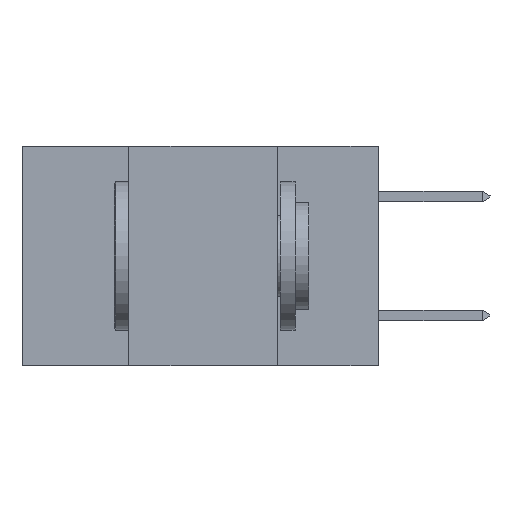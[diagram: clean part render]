
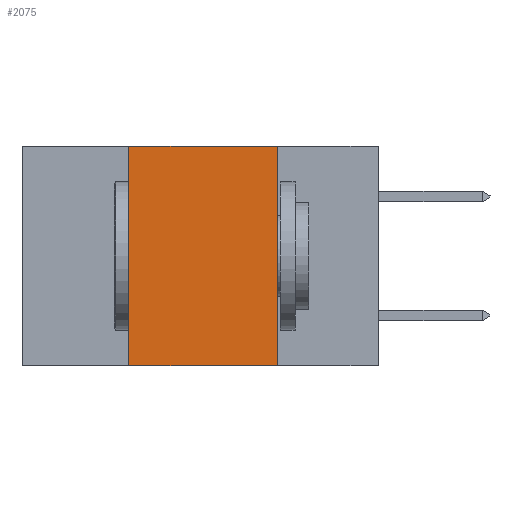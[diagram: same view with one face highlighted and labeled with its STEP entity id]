
A CAD part, left-side view. The second image highlights one B-rep face of the part: STEP entity #2075.
In plain terms, the highlighted planar face has unit normal (-1, 0, 0).
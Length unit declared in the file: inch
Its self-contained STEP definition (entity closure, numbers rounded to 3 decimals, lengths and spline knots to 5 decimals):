
#1141 = CARTESIAN_POINT ( 'NONE',  ( 0., 0.17, -0.37 ) ) ;
#2075 = ADVANCED_FACE ( 'NONE', ( #20528 ), #10109, .F. ) ;
#2426 = VECTOR ( 'NONE', #7298, 39.37008 ) ;
#3130 = CARTESIAN_POINT ( 'NONE',  ( 0., 0.6, 0. ) ) ;
#3871 = CARTESIAN_POINT ( 'NONE',  ( 0., 0.6, -0.37 ) ) ;
#3981 = LINE ( 'NONE', #3871, #6987 ) ;
#5074 = LINE ( 'NONE', #1141, #17252 ) ;
#5082 = LINE ( 'NONE', #11952, #12541 ) ;
#6987 = VECTOR ( 'NONE', #17351, 39.37008 ) ;
#7298 = DIRECTION ( 'NONE',  ( 0., -1., 0. ) ) ;
#7911 = ORIENTED_EDGE ( 'NONE', *, *, #15079, .T. ) ;
#8252 = CARTESIAN_POINT ( 'NONE',  ( 0., 0.42, -0.37 ) ) ;
#9280 = CARTESIAN_POINT ( 'NONE',  ( 0., 0.17, -0.37 ) ) ;
#9911 = CARTESIAN_POINT ( 'NONE',  ( 0., 0.42, 0. ) ) ;
#9912 = ORIENTED_EDGE ( 'NONE', *, *, #12412, .F. ) ;
#10005 = DIRECTION ( 'NONE',  ( 1., 0., 0. ) ) ;
#10109 = PLANE ( 'NONE',  #20768 ) ;
#10764 = VERTEX_POINT ( 'NONE', #8252 ) ;
#11936 = EDGE_CURVE ( 'NONE', #15763, #19973, #20974, .T. ) ;
#11952 = CARTESIAN_POINT ( 'NONE',  ( 0., 0.42, -0.37 ) ) ;
#12412 = EDGE_CURVE ( 'NONE', #19973, #20017, #5074, .T. ) ;
#12541 = VECTOR ( 'NONE', #18881, 39.37008 ) ;
#15079 = EDGE_CURVE ( 'NONE', #10764, #20017, #3981, .T. ) ;
#15763 = VERTEX_POINT ( 'NONE', #9911 ) ;
#16712 = DIRECTION ( 'NONE',  ( 0., 0., -1. ) ) ;
#16836 = ORIENTED_EDGE ( 'NONE', *, *, #16854, .F. ) ;
#16854 = EDGE_CURVE ( 'NONE', #10764, #15763, #5082, .T. ) ;
#17252 = VECTOR ( 'NONE', #20558, 39.37008 ) ;
#17351 = DIRECTION ( 'NONE',  ( 0., -1., 0. ) ) ;
#17620 = CARTESIAN_POINT ( 'NONE',  ( 0., 0.6, 0. ) ) ;
#17798 = CARTESIAN_POINT ( 'NONE',  ( 0., 0.17, 0. ) ) ;
#18144 = ORIENTED_EDGE ( 'NONE', *, *, #11936, .F. ) ;
#18881 = DIRECTION ( 'NONE',  ( 0., 0., 1. ) ) ;
#19973 = VERTEX_POINT ( 'NONE', #17798 ) ;
#20017 = VERTEX_POINT ( 'NONE', #9280 ) ;
#20528 = FACE_OUTER_BOUND ( 'NONE', #20686, .T. ) ;
#20558 = DIRECTION ( 'NONE',  ( 0., 0., -1. ) ) ;
#20686 = EDGE_LOOP ( 'NONE', ( #9912, #18144, #16836, #7911 ) ) ;
#20768 = AXIS2_PLACEMENT_3D ( 'NONE', #3130, #10005, #16712 ) ;
#20974 = LINE ( 'NONE', #17620, #2426 ) ;
